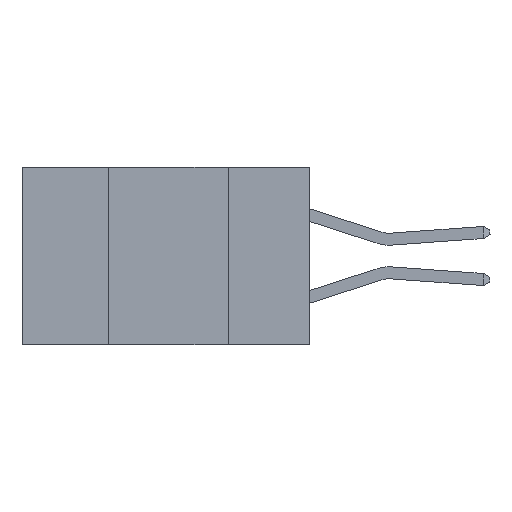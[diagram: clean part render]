
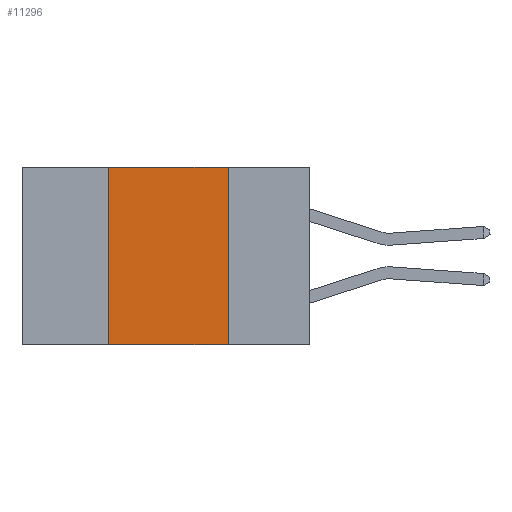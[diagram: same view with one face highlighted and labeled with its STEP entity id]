
A CAD part, left-side view. The second image highlights one B-rep face of the part: STEP entity #11296.
In plain terms, the highlighted planar face has unit normal (-1, 0, 0).
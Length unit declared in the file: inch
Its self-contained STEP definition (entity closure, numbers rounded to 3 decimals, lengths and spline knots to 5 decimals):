
#1684 = ORIENTED_EDGE ( 'NONE', *, *, #21264, .F. ) ;
#2022 = CARTESIAN_POINT ( 'NONE',  ( 0., 0.17, -0.37 ) ) ;
#3149 = DIRECTION ( 'NONE',  ( 1., 0., 0. ) ) ;
#3315 = LINE ( 'NONE', #6492, #17939 ) ;
#3361 = CARTESIAN_POINT ( 'NONE',  ( 0., 0.6, 0. ) ) ;
#3364 = LINE ( 'NONE', #8400, #3887 ) ;
#3839 = CARTESIAN_POINT ( 'NONE',  ( 0., 0.42, -0.37 ) ) ;
#3887 = VECTOR ( 'NONE', #14807, 39.37008 ) ;
#4070 = VERTEX_POINT ( 'NONE', #10785 ) ;
#4520 = ORIENTED_EDGE ( 'NONE', *, *, #6477, .T. ) ;
#5055 = EDGE_CURVE ( 'NONE', #9312, #15632, #6769, .T. ) ;
#5896 = EDGE_CURVE ( 'NONE', #15632, #6557, #3315, .T. ) ;
#6477 = EDGE_CURVE ( 'NONE', #4070, #6557, #3364, .T. ) ;
#6492 = CARTESIAN_POINT ( 'NONE',  ( 0., 0.17, -0.37 ) ) ;
#6557 = VERTEX_POINT ( 'NONE', #2022 ) ;
#6769 = LINE ( 'NONE', #3361, #9092 ) ;
#7992 = ORIENTED_EDGE ( 'NONE', *, *, #5055, .F. ) ;
#8196 = DIRECTION ( 'NONE',  ( 0., 0., -1. ) ) ;
#8400 = CARTESIAN_POINT ( 'NONE',  ( 0., 0.6, -0.37 ) ) ;
#8575 = ORIENTED_EDGE ( 'NONE', *, *, #5896, .F. ) ;
#9092 = VECTOR ( 'NONE', #10064, 39.37008 ) ;
#9312 = VERTEX_POINT ( 'NONE', #16480 ) ;
#10064 = DIRECTION ( 'NONE',  ( 0., -1., 0. ) ) ;
#10066 = CARTESIAN_POINT ( 'NONE',  ( 0., 0.6, 0. ) ) ;
#10785 = CARTESIAN_POINT ( 'NONE',  ( 0., 0.42, -0.37 ) ) ;
#11296 = ADVANCED_FACE ( 'NONE', ( #18232 ), #13253, .F. ) ;
#11902 = AXIS2_PLACEMENT_3D ( 'NONE', #10066, #3149, #8196 ) ;
#13253 = PLANE ( 'NONE',  #11902 ) ;
#13733 = LINE ( 'NONE', #3839, #21728 ) ;
#14807 = DIRECTION ( 'NONE',  ( 0., -1., 0. ) ) ;
#15632 = VERTEX_POINT ( 'NONE', #18965 ) ;
#16480 = CARTESIAN_POINT ( 'NONE',  ( 0., 0.42, 0. ) ) ;
#17939 = VECTOR ( 'NONE', #21704, 39.37008 ) ;
#18156 = EDGE_LOOP ( 'NONE', ( #8575, #7992, #1684, #4520 ) ) ;
#18232 = FACE_OUTER_BOUND ( 'NONE', #18156, .T. ) ;
#18965 = CARTESIAN_POINT ( 'NONE',  ( 0., 0.17, 0. ) ) ;
#20475 = DIRECTION ( 'NONE',  ( 0., 0., 1. ) ) ;
#21264 = EDGE_CURVE ( 'NONE', #4070, #9312, #13733, .T. ) ;
#21704 = DIRECTION ( 'NONE',  ( 0., 0., -1. ) ) ;
#21728 = VECTOR ( 'NONE', #20475, 39.37008 ) ;
